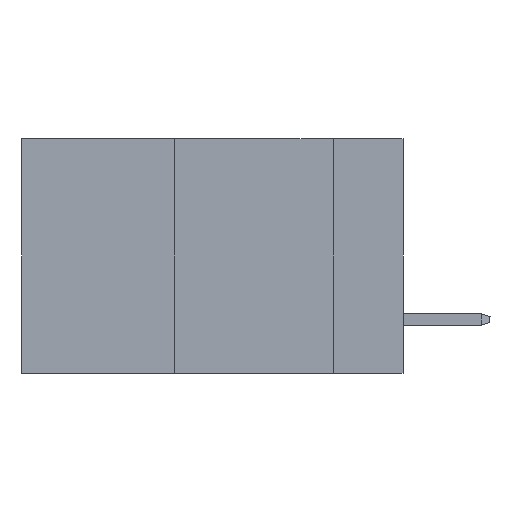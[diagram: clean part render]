
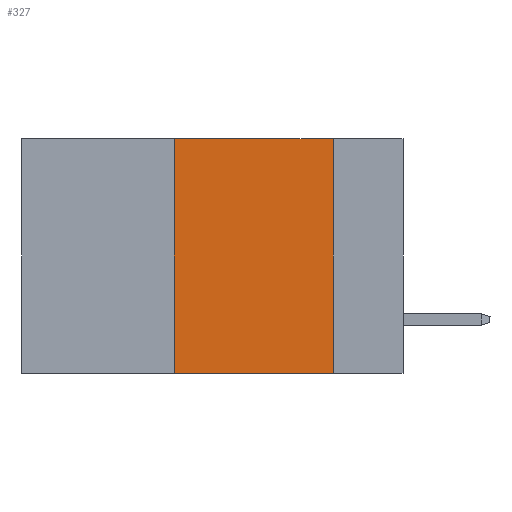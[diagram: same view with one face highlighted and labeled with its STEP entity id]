
A CAD part, left-side view. The second image highlights one B-rep face of the part: STEP entity #327.
In plain terms, the highlighted planar face has unit normal (-1, 0, 0).
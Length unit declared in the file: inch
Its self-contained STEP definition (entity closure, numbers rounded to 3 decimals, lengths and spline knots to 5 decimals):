
#327 = ADVANCED_FACE ( 'NONE', ( #21709 ), #18375, .F. ) ;
#671 = CARTESIAN_POINT ( 'NONE',  ( 0., 0.11, 0. ) ) ;
#1671 = CARTESIAN_POINT ( 'NONE',  ( 0., 0.36, 0. ) ) ;
#5169 = ORIENTED_EDGE ( 'NONE', *, *, #10740, .F. ) ;
#5320 = CARTESIAN_POINT ( 'NONE',  ( 0., 0.6, 0. ) ) ;
#6329 = ORIENTED_EDGE ( 'NONE', *, *, #17557, .F. ) ;
#6415 = VERTEX_POINT ( 'NONE', #671 ) ;
#8793 = VECTOR ( 'NONE', #13485, 39.37008 ) ;
#8912 = DIRECTION ( 'NONE',  ( 0., -1., 0. ) ) ;
#9173 = LINE ( 'NONE', #18542, #19632 ) ;
#9267 = ORIENTED_EDGE ( 'NONE', *, *, #9683, .T. ) ;
#9373 = ORIENTED_EDGE ( 'NONE', *, *, #16993, .F. ) ;
#9683 = EDGE_CURVE ( 'NONE', #14356, #13346, #19214, .T. ) ;
#10137 = LINE ( 'NONE', #13628, #24238 ) ;
#10740 = EDGE_CURVE ( 'NONE', #19148, #6415, #9173, .T. ) ;
#10912 = AXIS2_PLACEMENT_3D ( 'NONE', #5320, #23570, #23947 ) ;
#11838 = EDGE_LOOP ( 'NONE', ( #9373, #5169, #6329, #9267 ) ) ;
#13346 = VERTEX_POINT ( 'NONE', #14161 ) ;
#13485 = DIRECTION ( 'NONE',  ( 0., 0., -1. ) ) ;
#13592 = CARTESIAN_POINT ( 'NONE',  ( 0., 0.11, 0. ) ) ;
#13628 = CARTESIAN_POINT ( 'NONE',  ( 0., 0.36, 0. ) ) ;
#13674 = CARTESIAN_POINT ( 'NONE',  ( 0., 0.6, -0.37 ) ) ;
#14161 = CARTESIAN_POINT ( 'NONE',  ( 0., 0.11, -0.37 ) ) ;
#14300 = DIRECTION ( 'NONE',  ( 0., -1., 0. ) ) ;
#14356 = VERTEX_POINT ( 'NONE', #16178 ) ;
#16178 = CARTESIAN_POINT ( 'NONE',  ( 0., 0.36, -0.37 ) ) ;
#16993 = EDGE_CURVE ( 'NONE', #6415, #13346, #22849, .T. ) ;
#17557 = EDGE_CURVE ( 'NONE', #14356, #19148, #10137, .T. ) ;
#18375 = PLANE ( 'NONE',  #10912 ) ;
#18458 = VECTOR ( 'NONE', #14300, 39.37008 ) ;
#18542 = CARTESIAN_POINT ( 'NONE',  ( 0., 0.6, 0. ) ) ;
#19148 = VERTEX_POINT ( 'NONE', #1671 ) ;
#19214 = LINE ( 'NONE', #13674, #18458 ) ;
#19632 = VECTOR ( 'NONE', #8912, 39.37008 ) ;
#21122 = DIRECTION ( 'NONE',  ( 0., 0., 1. ) ) ;
#21709 = FACE_OUTER_BOUND ( 'NONE', #11838, .T. ) ;
#22849 = LINE ( 'NONE', #13592, #8793 ) ;
#23570 = DIRECTION ( 'NONE',  ( 1., 0., 0. ) ) ;
#23947 = DIRECTION ( 'NONE',  ( 0., 0., -1. ) ) ;
#24238 = VECTOR ( 'NONE', #21122, 39.37008 ) ;
